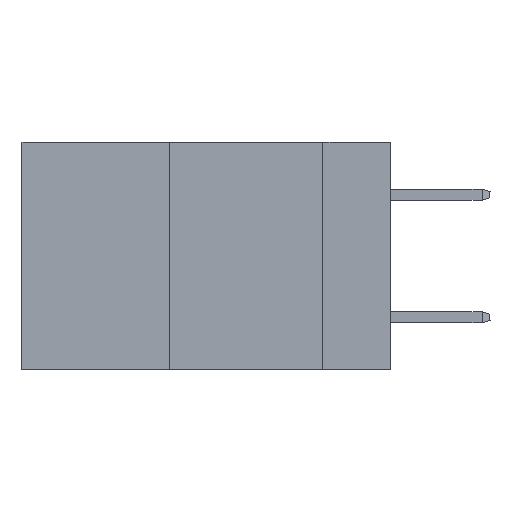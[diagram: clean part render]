
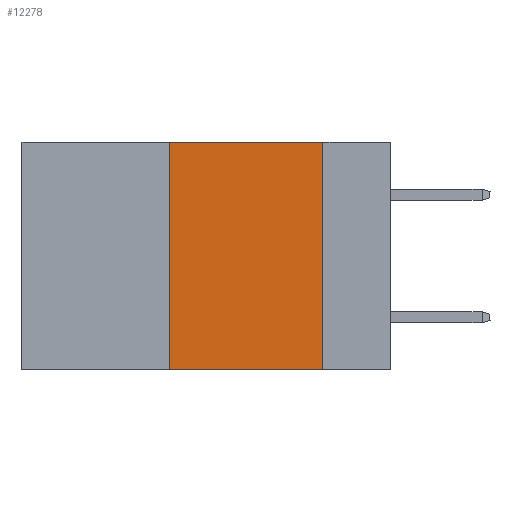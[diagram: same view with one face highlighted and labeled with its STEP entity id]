
A CAD part, left-side view. The second image highlights one B-rep face of the part: STEP entity #12278.
In plain terms, the highlighted planar face has unit normal (-1, 0, 0).
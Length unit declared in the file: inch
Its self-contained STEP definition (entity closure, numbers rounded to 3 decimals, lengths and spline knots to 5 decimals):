
#272 = LINE ( 'NONE', #4587, #23116 ) ;
#307 = DIRECTION ( 'NONE',  ( 0., 0., 1. ) ) ;
#470 = CARTESIAN_POINT ( 'NONE',  ( 0., 0.36, 0. ) ) ;
#906 = EDGE_CURVE ( 'NONE', #12916, #3567, #22867, .T. ) ;
#3567 = VERTEX_POINT ( 'NONE', #22288 ) ;
#3707 = VERTEX_POINT ( 'NONE', #13167 ) ;
#4587 = CARTESIAN_POINT ( 'NONE',  ( 0., 0.6, 0. ) ) ;
#4751 = ORIENTED_EDGE ( 'NONE', *, *, #16996, .F. ) ;
#6006 = EDGE_CURVE ( 'NONE', #3707, #19121, #272, .T. ) ;
#7619 = VECTOR ( 'NONE', #14392, 39.37008 ) ;
#8392 = CARTESIAN_POINT ( 'NONE',  ( 0., 0.11, 0. ) ) ;
#8418 = DIRECTION ( 'NONE',  ( 0., 0., -1. ) ) ;
#9776 = VECTOR ( 'NONE', #20555, 39.37008 ) ;
#10590 = VECTOR ( 'NONE', #307, 39.37008 ) ;
#11437 = ORIENTED_EDGE ( 'NONE', *, *, #21493, .F. ) ;
#11502 = CARTESIAN_POINT ( 'NONE',  ( 0., 0.11, 0. ) ) ;
#12278 = ADVANCED_FACE ( 'NONE', ( #12501 ), #17537, .F. ) ;
#12501 = FACE_OUTER_BOUND ( 'NONE', #12544, .T. ) ;
#12544 = EDGE_LOOP ( 'NONE', ( #11437, #17937, #4751, #14809 ) ) ;
#12916 = VERTEX_POINT ( 'NONE', #20238 ) ;
#13167 = CARTESIAN_POINT ( 'NONE',  ( 0., 0.36, 0. ) ) ;
#13655 = CARTESIAN_POINT ( 'NONE',  ( 0., 0.6, 0. ) ) ;
#13910 = LINE ( 'NONE', #470, #10590 ) ;
#14392 = DIRECTION ( 'NONE',  ( 0., -1., 0. ) ) ;
#14809 = ORIENTED_EDGE ( 'NONE', *, *, #906, .T. ) ;
#15684 = LINE ( 'NONE', #11502, #9776 ) ;
#16082 = CARTESIAN_POINT ( 'NONE',  ( 0., 0.6, -0.37 ) ) ;
#16996 = EDGE_CURVE ( 'NONE', #12916, #3707, #13910, .T. ) ;
#17385 = DIRECTION ( 'NONE',  ( 1., 0., 0. ) ) ;
#17537 = PLANE ( 'NONE',  #22916 ) ;
#17937 = ORIENTED_EDGE ( 'NONE', *, *, #6006, .F. ) ;
#18885 = DIRECTION ( 'NONE',  ( 0., -1., 0. ) ) ;
#19121 = VERTEX_POINT ( 'NONE', #8392 ) ;
#20238 = CARTESIAN_POINT ( 'NONE',  ( 0., 0.36, -0.37 ) ) ;
#20555 = DIRECTION ( 'NONE',  ( 0., 0., -1. ) ) ;
#21493 = EDGE_CURVE ( 'NONE', #19121, #3567, #15684, .T. ) ;
#22288 = CARTESIAN_POINT ( 'NONE',  ( 0., 0.11, -0.37 ) ) ;
#22867 = LINE ( 'NONE', #16082, #7619 ) ;
#22916 = AXIS2_PLACEMENT_3D ( 'NONE', #13655, #17385, #8418 ) ;
#23116 = VECTOR ( 'NONE', #18885, 39.37008 ) ;
